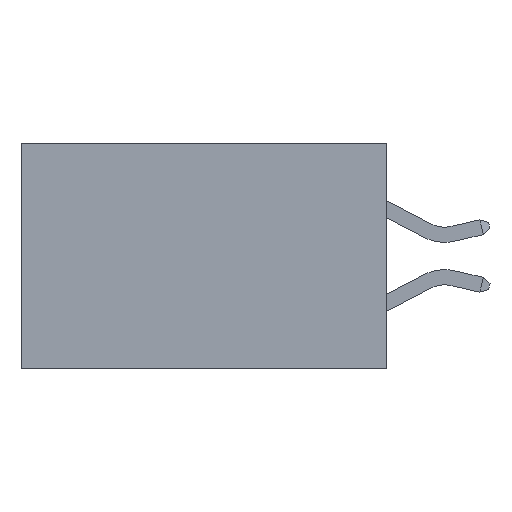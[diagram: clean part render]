
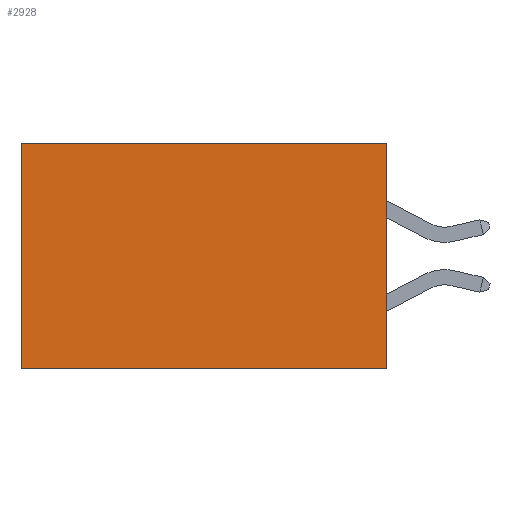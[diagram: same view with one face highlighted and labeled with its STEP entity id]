
A CAD part, left-side view. The second image highlights one B-rep face of the part: STEP entity #2928.
In plain terms, the highlighted planar face has unit normal (-1, 0, 0).
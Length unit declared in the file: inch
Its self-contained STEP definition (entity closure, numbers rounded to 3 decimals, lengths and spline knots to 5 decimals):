
#35 = EDGE_CURVE ( 'NONE', #12613, #13835, #1442, .T. ) ;
#1053 = DIRECTION ( 'NONE',  ( 0., 0., -1. ) ) ;
#1442 = LINE ( 'NONE', #7265, #7846 ) ;
#2309 = EDGE_LOOP ( 'NONE', ( #11963, #5620, #8187, #4251 ) ) ;
#2928 = ADVANCED_FACE ( 'NONE', ( #12220 ), #11201, .F. ) ;
#3444 = VERTEX_POINT ( 'NONE', #7154 ) ;
#4251 = ORIENTED_EDGE ( 'NONE', *, *, #10153, .T. ) ;
#4325 = LINE ( 'NONE', #5688, #10568 ) ;
#5369 = DIRECTION ( 'NONE',  ( 0., 1., 0. ) ) ;
#5620 = ORIENTED_EDGE ( 'NONE', *, *, #6746, .F. ) ;
#5688 = CARTESIAN_POINT ( 'NONE',  ( 0.2615, 0., 0. ) ) ;
#5797 = CARTESIAN_POINT ( 'NONE',  ( 0.2615, 0.6, 0. ) ) ;
#6746 = EDGE_CURVE ( 'NONE', #14735, #13835, #11037, .T. ) ;
#7154 = CARTESIAN_POINT ( 'NONE',  ( 0.2615, 0., 0. ) ) ;
#7265 = CARTESIAN_POINT ( 'NONE',  ( 0.2615, 0.6, -0.37 ) ) ;
#7459 = CARTESIAN_POINT ( 'NONE',  ( 0.2615, 0., -0.37 ) ) ;
#7846 = VECTOR ( 'NONE', #14190, 39.37008 ) ;
#8187 = ORIENTED_EDGE ( 'NONE', *, *, #11476, .F. ) ;
#10120 = VECTOR ( 'NONE', #1053, 39.37008 ) ;
#10153 = EDGE_CURVE ( 'NONE', #3444, #12613, #4325, .T. ) ;
#10568 = VECTOR ( 'NONE', #5369, 39.37008 ) ;
#11037 = LINE ( 'NONE', #15324, #13935 ) ;
#11142 = DIRECTION ( 'NONE',  ( 0., 0., -1. ) ) ;
#11154 = DIRECTION ( 'NONE',  ( 1., 0., 0. ) ) ;
#11177 = CARTESIAN_POINT ( 'NONE',  ( 0.2615, 0., -0.37 ) ) ;
#11201 = PLANE ( 'NONE',  #13981 ) ;
#11355 = CARTESIAN_POINT ( 'NONE',  ( 0.2615, 0.6, -0.37 ) ) ;
#11476 = EDGE_CURVE ( 'NONE', #3444, #14735, #13409, .T. ) ;
#11963 = ORIENTED_EDGE ( 'NONE', *, *, #35, .T. ) ;
#12220 = FACE_OUTER_BOUND ( 'NONE', #2309, .T. ) ;
#12613 = VERTEX_POINT ( 'NONE', #5797 ) ;
#13409 = LINE ( 'NONE', #7459, #10120 ) ;
#13835 = VERTEX_POINT ( 'NONE', #11355 ) ;
#13935 = VECTOR ( 'NONE', #16149, 39.37008 ) ;
#13981 = AXIS2_PLACEMENT_3D ( 'NONE', #11177, #11154, #11142 ) ;
#14190 = DIRECTION ( 'NONE',  ( 0., 0., -1. ) ) ;
#14735 = VERTEX_POINT ( 'NONE', #15413 ) ;
#15324 = CARTESIAN_POINT ( 'NONE',  ( 0.2615, 0., -0.37 ) ) ;
#15413 = CARTESIAN_POINT ( 'NONE',  ( 0.2615, 0., -0.37 ) ) ;
#16149 = DIRECTION ( 'NONE',  ( 0., 1., 0. ) ) ;
